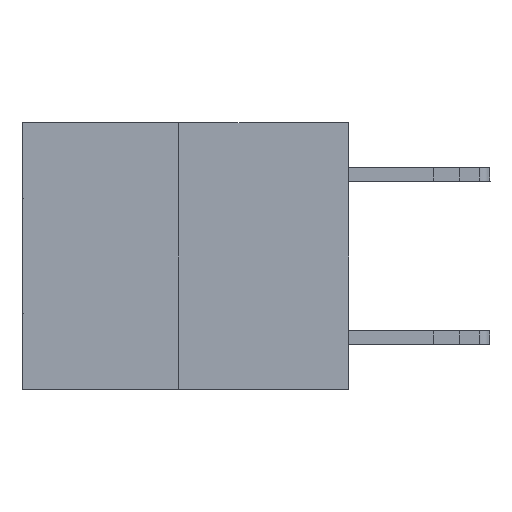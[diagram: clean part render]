
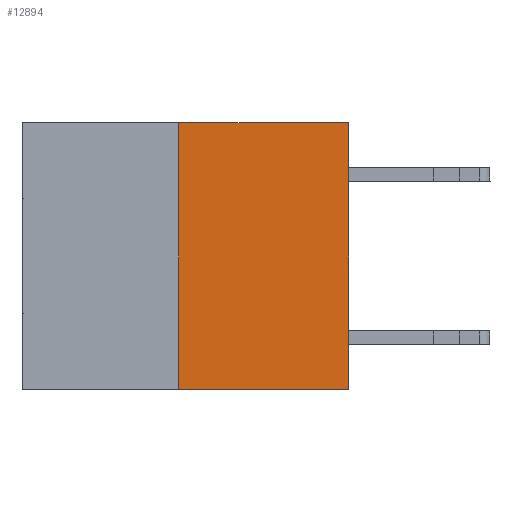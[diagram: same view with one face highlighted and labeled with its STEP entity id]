
A CAD part, left-side view. The second image highlights one B-rep face of the part: STEP entity #12894.
In plain terms, the highlighted planar face has unit normal (-1, 0, 0).
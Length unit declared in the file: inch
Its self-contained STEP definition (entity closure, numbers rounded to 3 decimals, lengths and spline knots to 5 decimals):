
#656 = ORIENTED_EDGE ( 'NONE', *, *, #3301, .T. ) ;
#1627 = VERTEX_POINT ( 'NONE', #10315 ) ;
#2320 = CARTESIAN_POINT ( 'NONE',  ( 0., 0., 0. ) ) ;
#2982 = LINE ( 'NONE', #2320, #33131 ) ;
#3301 = EDGE_CURVE ( 'NONE', #1627, #16943, #2982, .T. ) ;
#5194 = VECTOR ( 'NONE', #7077, 39.37008 ) ;
#5608 = LINE ( 'NONE', #9988, #5194 ) ;
#6457 = VERTEX_POINT ( 'NONE', #18825 ) ;
#7077 = DIRECTION ( 'NONE',  ( 0., 0., 1. ) ) ;
#8383 = DIRECTION ( 'NONE',  ( 0., -1., 0. ) ) ;
#9988 = CARTESIAN_POINT ( 'NONE',  ( 0., 0.312, -0.49 ) ) ;
#10233 = DIRECTION ( 'NONE',  ( 0., 0., -1. ) ) ;
#10315 = CARTESIAN_POINT ( 'NONE',  ( 0., 0., -0.49 ) ) ;
#11092 = CARTESIAN_POINT ( 'NONE',  ( 0., 0.6, -0.49 ) ) ;
#11998 = CARTESIAN_POINT ( 'NONE',  ( 0., 0.6, 0. ) ) ;
#12152 = VECTOR ( 'NONE', #8383, 39.37008 ) ;
#12207 = FACE_OUTER_BOUND ( 'NONE', #28680, .T. ) ;
#12894 = ADVANCED_FACE ( 'NONE', ( #12207 ), #23435, .F. ) ;
#15225 = VERTEX_POINT ( 'NONE', #28948 ) ;
#15600 = AXIS2_PLACEMENT_3D ( 'NONE', #22987, #25560, #10233 ) ;
#16943 = VERTEX_POINT ( 'NONE', #32461 ) ;
#17605 = VECTOR ( 'NONE', #24962, 39.37008 ) ;
#17843 = ORIENTED_EDGE ( 'NONE', *, *, #21770, .F. ) ;
#18825 = CARTESIAN_POINT ( 'NONE',  ( 0., 0.312, -0.49 ) ) ;
#19785 = EDGE_CURVE ( 'NONE', #6457, #1627, #30177, .T. ) ;
#21188 = EDGE_CURVE ( 'NONE', #6457, #15225, #5608, .T. ) ;
#21770 = EDGE_CURVE ( 'NONE', #15225, #16943, #21986, .T. ) ;
#21986 = LINE ( 'NONE', #11998, #17605 ) ;
#22524 = DIRECTION ( 'NONE',  ( 0., 0., 1. ) ) ;
#22987 = CARTESIAN_POINT ( 'NONE',  ( 0., 0.6, 0. ) ) ;
#23435 = PLANE ( 'NONE',  #15600 ) ;
#24962 = DIRECTION ( 'NONE',  ( 0., -1., 0. ) ) ;
#25560 = DIRECTION ( 'NONE',  ( 1., 0., 0. ) ) ;
#28680 = EDGE_LOOP ( 'NONE', ( #32963, #28772, #656, #17843 ) ) ;
#28772 = ORIENTED_EDGE ( 'NONE', *, *, #19785, .T. ) ;
#28948 = CARTESIAN_POINT ( 'NONE',  ( 0., 0.312, 0. ) ) ;
#30177 = LINE ( 'NONE', #11092, #12152 ) ;
#32461 = CARTESIAN_POINT ( 'NONE',  ( 0., 0., 0. ) ) ;
#32963 = ORIENTED_EDGE ( 'NONE', *, *, #21188, .F. ) ;
#33131 = VECTOR ( 'NONE', #22524, 39.37008 ) ;
